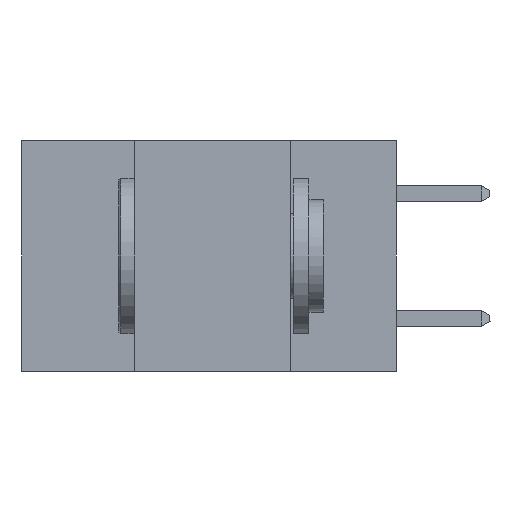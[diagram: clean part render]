
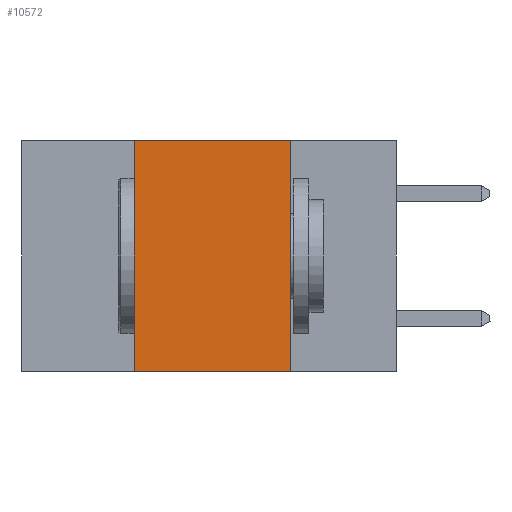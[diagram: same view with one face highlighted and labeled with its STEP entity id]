
A CAD part, left-side view. The second image highlights one B-rep face of the part: STEP entity #10572.
In plain terms, the highlighted planar face has unit normal (-1, 0, 0).
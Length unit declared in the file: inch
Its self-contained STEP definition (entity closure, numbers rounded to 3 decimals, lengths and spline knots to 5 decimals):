
#356 = LINE ( 'NONE', #3088, #17711 ) ;
#612 = DIRECTION ( 'NONE',  ( 0., 0., 1. ) ) ;
#883 = DIRECTION ( 'NONE',  ( 0., 0., -1. ) ) ;
#3088 = CARTESIAN_POINT ( 'NONE',  ( 0., 0.6, -0.37 ) ) ;
#3421 = ORIENTED_EDGE ( 'NONE', *, *, #24916, .T. ) ;
#3502 = VERTEX_POINT ( 'NONE', #16009 ) ;
#4092 = ORIENTED_EDGE ( 'NONE', *, *, #5065, .F. ) ;
#4796 = CARTESIAN_POINT ( 'NONE',  ( 0., 0.6, 0. ) ) ;
#5065 = EDGE_CURVE ( 'NONE', #5408, #5456, #23131, .T. ) ;
#5408 = VERTEX_POINT ( 'NONE', #16551 ) ;
#5456 = VERTEX_POINT ( 'NONE', #22749 ) ;
#5995 = VECTOR ( 'NONE', #17911, 39.37008 ) ;
#6530 = EDGE_CURVE ( 'NONE', #5456, #3502, #8044, .T. ) ;
#8030 = VERTEX_POINT ( 'NONE', #15339 ) ;
#8044 = LINE ( 'NONE', #19958, #5995 ) ;
#8137 = EDGE_LOOP ( 'NONE', ( #11157, #4092, #14618, #3421 ) ) ;
#10572 = ADVANCED_FACE ( 'NONE', ( #13246 ), #13486, .F. ) ;
#11157 = ORIENTED_EDGE ( 'NONE', *, *, #6530, .F. ) ;
#13246 = FACE_OUTER_BOUND ( 'NONE', #8137, .T. ) ;
#13486 = PLANE ( 'NONE',  #26362 ) ;
#13576 = DIRECTION ( 'NONE',  ( 1., 0., 0. ) ) ;
#13717 = DIRECTION ( 'NONE',  ( 0., -1., 0. ) ) ;
#13761 = LINE ( 'NONE', #25473, #23912 ) ;
#14618 = ORIENTED_EDGE ( 'NONE', *, *, #19480, .F. ) ;
#15339 = CARTESIAN_POINT ( 'NONE',  ( 0., 0.42, -0.37 ) ) ;
#16009 = CARTESIAN_POINT ( 'NONE',  ( 0., 0.17, -0.37 ) ) ;
#16551 = CARTESIAN_POINT ( 'NONE',  ( 0., 0.42, 0. ) ) ;
#17711 = VECTOR ( 'NONE', #13717, 39.37008 ) ;
#17911 = DIRECTION ( 'NONE',  ( 0., 0., -1. ) ) ;
#19480 = EDGE_CURVE ( 'NONE', #8030, #5408, #13761, .T. ) ;
#19600 = CARTESIAN_POINT ( 'NONE',  ( 0., 0.6, 0. ) ) ;
#19958 = CARTESIAN_POINT ( 'NONE',  ( 0., 0.17, -0.37 ) ) ;
#21351 = DIRECTION ( 'NONE',  ( 0., -1., 0. ) ) ;
#22480 = VECTOR ( 'NONE', #21351, 39.37008 ) ;
#22749 = CARTESIAN_POINT ( 'NONE',  ( 0., 0.17, 0. ) ) ;
#23131 = LINE ( 'NONE', #4796, #22480 ) ;
#23912 = VECTOR ( 'NONE', #612, 39.37008 ) ;
#24916 = EDGE_CURVE ( 'NONE', #8030, #3502, #356, .T. ) ;
#25473 = CARTESIAN_POINT ( 'NONE',  ( 0., 0.42, -0.37 ) ) ;
#26362 = AXIS2_PLACEMENT_3D ( 'NONE', #19600, #13576, #883 ) ;
